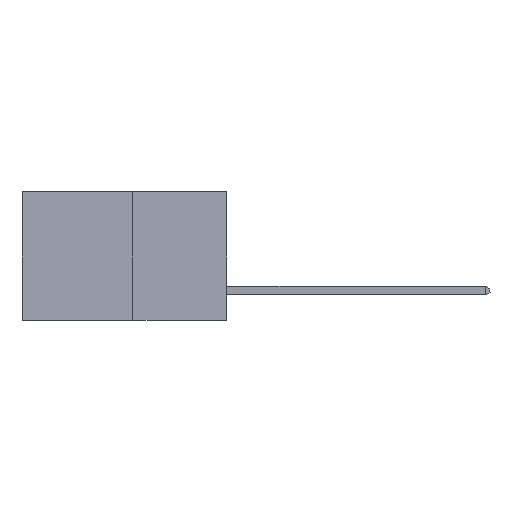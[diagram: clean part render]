
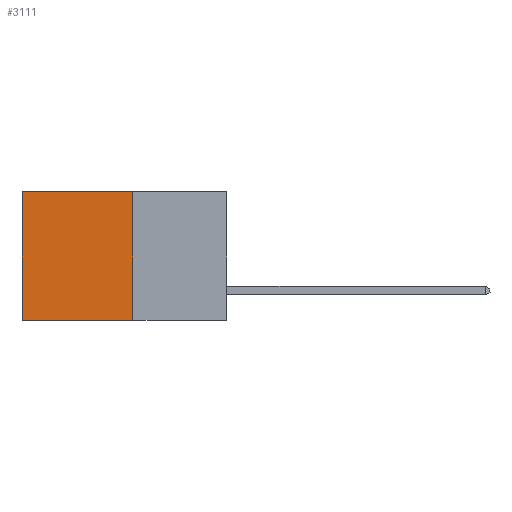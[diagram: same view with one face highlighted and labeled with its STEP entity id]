
A CAD part, left-side view. The second image highlights one B-rep face of the part: STEP entity #3111.
In plain terms, the highlighted planar face has unit normal (-1, 0, 0).
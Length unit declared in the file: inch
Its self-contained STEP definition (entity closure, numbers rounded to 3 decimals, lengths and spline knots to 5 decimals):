
#465 = LINE ( 'NONE', #10364, #1200 ) ;
#910 = CARTESIAN_POINT ( 'NONE',  ( 0.277, 0.59, 0. ) ) ;
#1200 = VECTOR ( 'NONE', #5678, 39.37008 ) ;
#1517 = EDGE_CURVE ( 'NONE', #24363, #18345, #26349, .T. ) ;
#1842 = DIRECTION ( 'NONE',  ( 1., 0., 0. ) ) ;
#2951 = EDGE_LOOP ( 'NONE', ( #20850, #22826, #9090, #8936 ) ) ;
#3111 = ADVANCED_FACE ( 'NONE', ( #4768 ), #22580, .F. ) ;
#3202 = LINE ( 'NONE', #3466, #27757 ) ;
#3324 = VECTOR ( 'NONE', #22719, 39.37008 ) ;
#3466 = CARTESIAN_POINT ( 'NONE',  ( 0.277, 0.27, -0.37 ) ) ;
#4768 = FACE_OUTER_BOUND ( 'NONE', #2951, .T. ) ;
#5678 = DIRECTION ( 'NONE',  ( 0., 0., -1. ) ) ;
#6863 = CARTESIAN_POINT ( 'NONE',  ( 0.277, 0.27, 0. ) ) ;
#8922 = CARTESIAN_POINT ( 'NONE',  ( 0.277, 0.27, -0.37 ) ) ;
#8936 = ORIENTED_EDGE ( 'NONE', *, *, #1517, .T. ) ;
#9090 = ORIENTED_EDGE ( 'NONE', *, *, #13764, .F. ) ;
#10085 = CARTESIAN_POINT ( 'NONE',  ( 0.277, 0.59, -0.37 ) ) ;
#10364 = CARTESIAN_POINT ( 'NONE',  ( 0.277, 0.59, -0.37 ) ) ;
#11102 = CARTESIAN_POINT ( 'NONE',  ( 0.277, 0.27, -0.37 ) ) ;
#13764 = EDGE_CURVE ( 'NONE', #24363, #27132, #15657, .T. ) ;
#15657 = LINE ( 'NONE', #8922, #3324 ) ;
#17162 = EDGE_CURVE ( 'NONE', #27132, #20230, #3202, .T. ) ;
#18062 = DIRECTION ( 'NONE',  ( 0., 0., -1. ) ) ;
#18345 = VERTEX_POINT ( 'NONE', #910 ) ;
#19667 = DIRECTION ( 'NONE',  ( 0., 1., 0. ) ) ;
#20230 = VERTEX_POINT ( 'NONE', #10085 ) ;
#20231 = VECTOR ( 'NONE', #25209, 39.37008 ) ;
#20306 = EDGE_CURVE ( 'NONE', #18345, #20230, #465, .T. ) ;
#20850 = ORIENTED_EDGE ( 'NONE', *, *, #20306, .T. ) ;
#22261 = CARTESIAN_POINT ( 'NONE',  ( 0.277, 0.27, -0.37 ) ) ;
#22580 = PLANE ( 'NONE',  #22629 ) ;
#22629 = AXIS2_PLACEMENT_3D ( 'NONE', #11102, #1842, #18062 ) ;
#22719 = DIRECTION ( 'NONE',  ( 0., 0., -1. ) ) ;
#22826 = ORIENTED_EDGE ( 'NONE', *, *, #17162, .F. ) ;
#24363 = VERTEX_POINT ( 'NONE', #28529 ) ;
#25209 = DIRECTION ( 'NONE',  ( 0., 1., 0. ) ) ;
#26349 = LINE ( 'NONE', #6863, #20231 ) ;
#27132 = VERTEX_POINT ( 'NONE', #22261 ) ;
#27757 = VECTOR ( 'NONE', #19667, 39.37008 ) ;
#28529 = CARTESIAN_POINT ( 'NONE',  ( 0.277, 0.27, 0. ) ) ;
